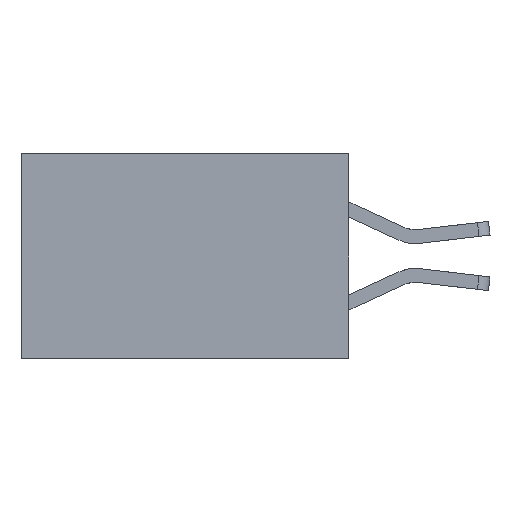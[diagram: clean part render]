
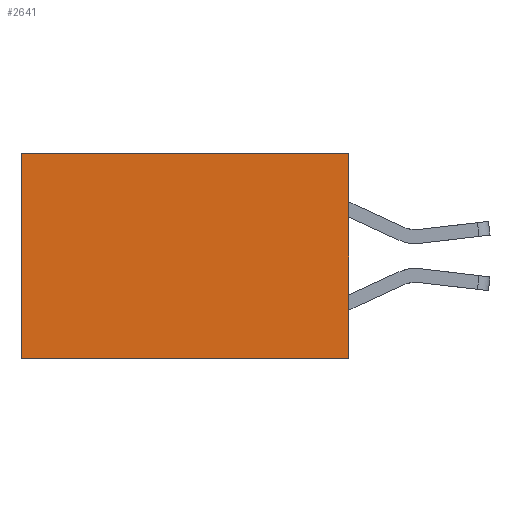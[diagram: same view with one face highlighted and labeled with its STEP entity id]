
A CAD part, left-side view. The second image highlights one B-rep face of the part: STEP entity #2641.
In plain terms, the highlighted planar face has unit normal (-1, 0, 0).
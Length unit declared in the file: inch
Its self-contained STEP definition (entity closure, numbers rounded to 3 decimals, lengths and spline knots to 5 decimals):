
#327 = DIRECTION ( 'NONE',  ( 0., 1., 0. ) ) ;
#335 = VERTEX_POINT ( 'NONE', #11839 ) ;
#595 = CARTESIAN_POINT ( 'NONE',  ( 0.277, 0.59, -0.37 ) ) ;
#1200 = CARTESIAN_POINT ( 'NONE',  ( 0.277, 0.59, 0. ) ) ;
#1415 = VECTOR ( 'NONE', #7269, 39.37008 ) ;
#2081 = LINE ( 'NONE', #6265, #10714 ) ;
#2641 = ADVANCED_FACE ( 'NONE', ( #7713 ), #13286, .F. ) ;
#3176 = LINE ( 'NONE', #14862, #15486 ) ;
#3365 = EDGE_CURVE ( 'NONE', #7294, #13684, #2081, .T. ) ;
#4821 = LINE ( 'NONE', #6074, #1415 ) ;
#5196 = EDGE_LOOP ( 'NONE', ( #9458, #10561, #7658, #11232 ) ) ;
#6074 = CARTESIAN_POINT ( 'NONE',  ( 0.277, 0., -0.37 ) ) ;
#6265 = CARTESIAN_POINT ( 'NONE',  ( 0.277, 0., -0.37 ) ) ;
#7269 = DIRECTION ( 'NONE',  ( 0., 0., -1. ) ) ;
#7294 = VERTEX_POINT ( 'NONE', #11048 ) ;
#7658 = ORIENTED_EDGE ( 'NONE', *, *, #11607, .F. ) ;
#7713 = FACE_OUTER_BOUND ( 'NONE', #5196, .T. ) ;
#8474 = VERTEX_POINT ( 'NONE', #1200 ) ;
#9217 = DIRECTION ( 'NONE',  ( 0., 0., -1. ) ) ;
#9458 = ORIENTED_EDGE ( 'NONE', *, *, #15403, .T. ) ;
#10561 = ORIENTED_EDGE ( 'NONE', *, *, #3365, .F. ) ;
#10714 = VECTOR ( 'NONE', #12988, 39.37008 ) ;
#11048 = CARTESIAN_POINT ( 'NONE',  ( 0.277, 0., -0.37 ) ) ;
#11232 = ORIENTED_EDGE ( 'NONE', *, *, #13471, .T. ) ;
#11607 = EDGE_CURVE ( 'NONE', #335, #7294, #4821, .T. ) ;
#11762 = DIRECTION ( 'NONE',  ( 0., 0., -1. ) ) ;
#11839 = CARTESIAN_POINT ( 'NONE',  ( 0.277, 0., 0. ) ) ;
#12988 = DIRECTION ( 'NONE',  ( 0., 1., 0. ) ) ;
#13126 = AXIS2_PLACEMENT_3D ( 'NONE', #13242, #13300, #11762 ) ;
#13242 = CARTESIAN_POINT ( 'NONE',  ( 0.277, 0., -0.37 ) ) ;
#13286 = PLANE ( 'NONE',  #13126 ) ;
#13300 = DIRECTION ( 'NONE',  ( 1., 0., 0. ) ) ;
#13468 = LINE ( 'NONE', #595, #13845 ) ;
#13471 = EDGE_CURVE ( 'NONE', #335, #8474, #3176, .T. ) ;
#13684 = VERTEX_POINT ( 'NONE', #14124 ) ;
#13845 = VECTOR ( 'NONE', #9217, 39.37008 ) ;
#14124 = CARTESIAN_POINT ( 'NONE',  ( 0.277, 0.59, -0.37 ) ) ;
#14862 = CARTESIAN_POINT ( 'NONE',  ( 0.277, 0., 0. ) ) ;
#15403 = EDGE_CURVE ( 'NONE', #8474, #13684, #13468, .T. ) ;
#15486 = VECTOR ( 'NONE', #327, 39.37008 ) ;
